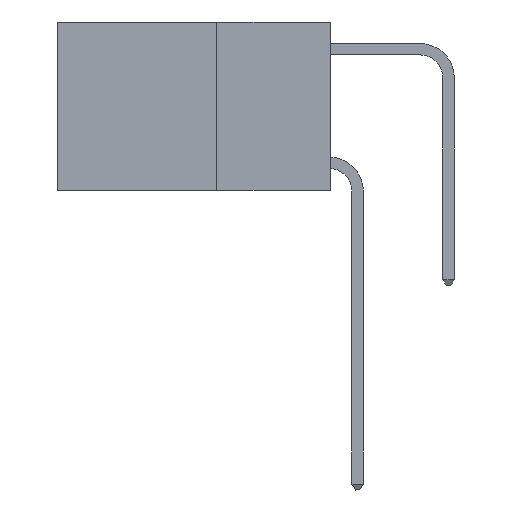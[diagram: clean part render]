
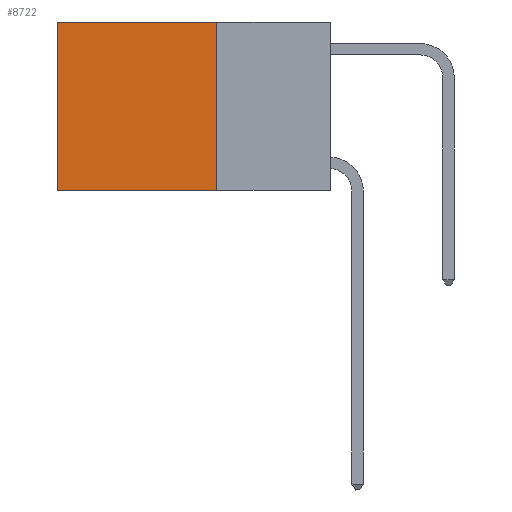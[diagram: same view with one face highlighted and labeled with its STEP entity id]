
A CAD part, left-side view. The second image highlights one B-rep face of the part: STEP entity #8722.
In plain terms, the highlighted planar face has unit normal (-1, 0, 0).
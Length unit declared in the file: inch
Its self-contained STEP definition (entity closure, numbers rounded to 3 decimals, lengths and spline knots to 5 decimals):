
#506 = CARTESIAN_POINT ( 'NONE',  ( 0.2625, 0.25, 0. ) ) ;
#904 = LINE ( 'NONE', #22345, #2135 ) ;
#1914 = LINE ( 'NONE', #7396, #14459 ) ;
#2135 = VECTOR ( 'NONE', #12127, 39.37008 ) ;
#3060 = CARTESIAN_POINT ( 'NONE',  ( 0.2625, 0.6, -0.37 ) ) ;
#4260 = CARTESIAN_POINT ( 'NONE',  ( 0.2625, 0.25, 0. ) ) ;
#4696 = ORIENTED_EDGE ( 'NONE', *, *, #10490, .T. ) ;
#5294 = VERTEX_POINT ( 'NONE', #8922 ) ;
#5662 = EDGE_CURVE ( 'NONE', #22038, #9782, #904, .T. ) ;
#6610 = VECTOR ( 'NONE', #22589, 39.37008 ) ;
#7396 = CARTESIAN_POINT ( 'NONE',  ( 0.2625, 0.25, -0.37 ) ) ;
#7595 = EDGE_CURVE ( 'NONE', #5294, #9782, #1914, .T. ) ;
#7873 = DIRECTION ( 'NONE',  ( 0., 0., -1. ) ) ;
#8722 = ADVANCED_FACE ( 'NONE', ( #20245 ), #20477, .F. ) ;
#8922 = CARTESIAN_POINT ( 'NONE',  ( 0.2625, 0.25, -0.37 ) ) ;
#9694 = DIRECTION ( 'NONE',  ( 1., 0., 0. ) ) ;
#9782 = VERTEX_POINT ( 'NONE', #3060 ) ;
#10490 = EDGE_CURVE ( 'NONE', #10787, #22038, #18126, .T. ) ;
#10787 = VERTEX_POINT ( 'NONE', #21120 ) ;
#11780 = CARTESIAN_POINT ( 'NONE',  ( 0.2625, 0.6, 0. ) ) ;
#12127 = DIRECTION ( 'NONE',  ( 0., 0., -1. ) ) ;
#12691 = AXIS2_PLACEMENT_3D ( 'NONE', #4260, #9694, #7873 ) ;
#12701 = ORIENTED_EDGE ( 'NONE', *, *, #7595, .F. ) ;
#14007 = ORIENTED_EDGE ( 'NONE', *, *, #5662, .T. ) ;
#14192 = DIRECTION ( 'NONE',  ( 0., 1., 0. ) ) ;
#14459 = VECTOR ( 'NONE', #22763, 39.37008 ) ;
#15602 = ORIENTED_EDGE ( 'NONE', *, *, #21135, .F. ) ;
#18126 = LINE ( 'NONE', #506, #21598 ) ;
#18360 = EDGE_LOOP ( 'NONE', ( #14007, #12701, #15602, #4696 ) ) ;
#18680 = LINE ( 'NONE', #18913, #6610 ) ;
#18913 = CARTESIAN_POINT ( 'NONE',  ( 0.2625, 0.25, 0. ) ) ;
#20245 = FACE_OUTER_BOUND ( 'NONE', #18360, .T. ) ;
#20477 = PLANE ( 'NONE',  #12691 ) ;
#21120 = CARTESIAN_POINT ( 'NONE',  ( 0.2625, 0.25, 0. ) ) ;
#21135 = EDGE_CURVE ( 'NONE', #10787, #5294, #18680, .T. ) ;
#21598 = VECTOR ( 'NONE', #14192, 39.37008 ) ;
#22038 = VERTEX_POINT ( 'NONE', #11780 ) ;
#22345 = CARTESIAN_POINT ( 'NONE',  ( 0.2625, 0.6, 0. ) ) ;
#22589 = DIRECTION ( 'NONE',  ( 0., 0., -1. ) ) ;
#22763 = DIRECTION ( 'NONE',  ( 0., 1., 0. ) ) ;
